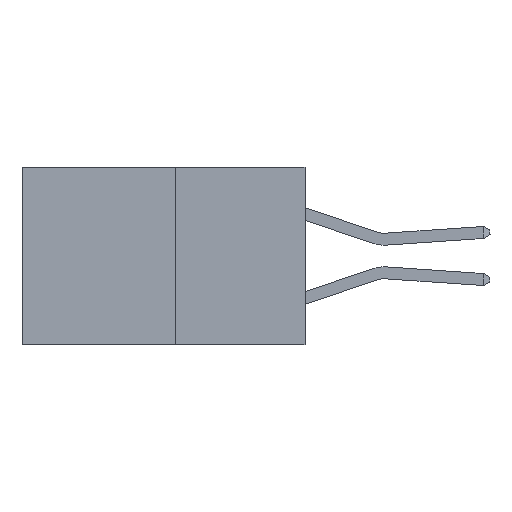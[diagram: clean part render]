
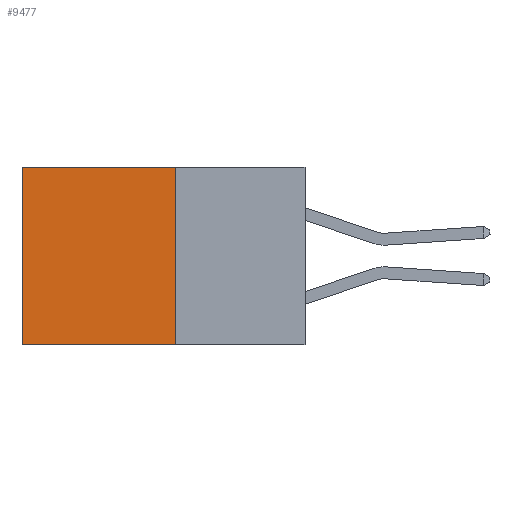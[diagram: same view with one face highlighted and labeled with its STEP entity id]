
A CAD part, left-side view. The second image highlights one B-rep face of the part: STEP entity #9477.
In plain terms, the highlighted planar face has unit normal (-1, 0, 0).
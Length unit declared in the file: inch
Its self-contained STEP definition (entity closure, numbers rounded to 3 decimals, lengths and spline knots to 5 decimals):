
#110 = EDGE_CURVE ( 'NONE', #5270, #5255, #8396, .T. ) ;
#227 = DIRECTION ( 'NONE',  ( 0., 0., -1. ) ) ;
#308 = CARTESIAN_POINT ( 'NONE',  ( 0.277, 0.27, -0.37 ) ) ;
#1463 = CARTESIAN_POINT ( 'NONE',  ( 0.277, 0.59, -0.37 ) ) ;
#1963 = ORIENTED_EDGE ( 'NONE', *, *, #6456, .F. ) ;
#3447 = EDGE_LOOP ( 'NONE', ( #4164, #1963, #6608, #6298 ) ) ;
#3464 = DIRECTION ( 'NONE',  ( 1., 0., 0. ) ) ;
#4164 = ORIENTED_EDGE ( 'NONE', *, *, #110, .T. ) ;
#4529 = VECTOR ( 'NONE', #5404, 39.37008 ) ;
#4831 = CARTESIAN_POINT ( 'NONE',  ( 0.277, 0.27, 0. ) ) ;
#4897 = DIRECTION ( 'NONE',  ( 0., 1., 0. ) ) ;
#4943 = VERTEX_POINT ( 'NONE', #4831 ) ;
#4967 = CARTESIAN_POINT ( 'NONE',  ( 0.277, 0.27, -0.37 ) ) ;
#5255 = VERTEX_POINT ( 'NONE', #1463 ) ;
#5270 = VERTEX_POINT ( 'NONE', #6034 ) ;
#5404 = DIRECTION ( 'NONE',  ( 0., 1., 0. ) ) ;
#5415 = CARTESIAN_POINT ( 'NONE',  ( 0.277, 0.27, 0. ) ) ;
#5609 = LINE ( 'NONE', #4967, #9891 ) ;
#5968 = VERTEX_POINT ( 'NONE', #9053 ) ;
#6034 = CARTESIAN_POINT ( 'NONE',  ( 0.277, 0.59, 0. ) ) ;
#6051 = VECTOR ( 'NONE', #11147, 39.37008 ) ;
#6298 = ORIENTED_EDGE ( 'NONE', *, *, #8494, .T. ) ;
#6456 = EDGE_CURVE ( 'NONE', #5968, #5255, #5609, .T. ) ;
#6608 = ORIENTED_EDGE ( 'NONE', *, *, #6909, .F. ) ;
#6909 = EDGE_CURVE ( 'NONE', #4943, #5968, #10129, .T. ) ;
#7184 = AXIS2_PLACEMENT_3D ( 'NONE', #8609, #3464, #9460 ) ;
#7947 = VECTOR ( 'NONE', #227, 39.37008 ) ;
#8396 = LINE ( 'NONE', #10018, #6051 ) ;
#8494 = EDGE_CURVE ( 'NONE', #4943, #5270, #10983, .T. ) ;
#8609 = CARTESIAN_POINT ( 'NONE',  ( 0.277, 0.27, -0.37 ) ) ;
#8646 = PLANE ( 'NONE',  #7184 ) ;
#9053 = CARTESIAN_POINT ( 'NONE',  ( 0.277, 0.27, -0.37 ) ) ;
#9460 = DIRECTION ( 'NONE',  ( 0., 0., -1. ) ) ;
#9477 = ADVANCED_FACE ( 'NONE', ( #10206 ), #8646, .F. ) ;
#9891 = VECTOR ( 'NONE', #4897, 39.37008 ) ;
#10018 = CARTESIAN_POINT ( 'NONE',  ( 0.277, 0.59, -0.37 ) ) ;
#10129 = LINE ( 'NONE', #308, #7947 ) ;
#10206 = FACE_OUTER_BOUND ( 'NONE', #3447, .T. ) ;
#10983 = LINE ( 'NONE', #5415, #4529 ) ;
#11147 = DIRECTION ( 'NONE',  ( 0., 0., -1. ) ) ;
